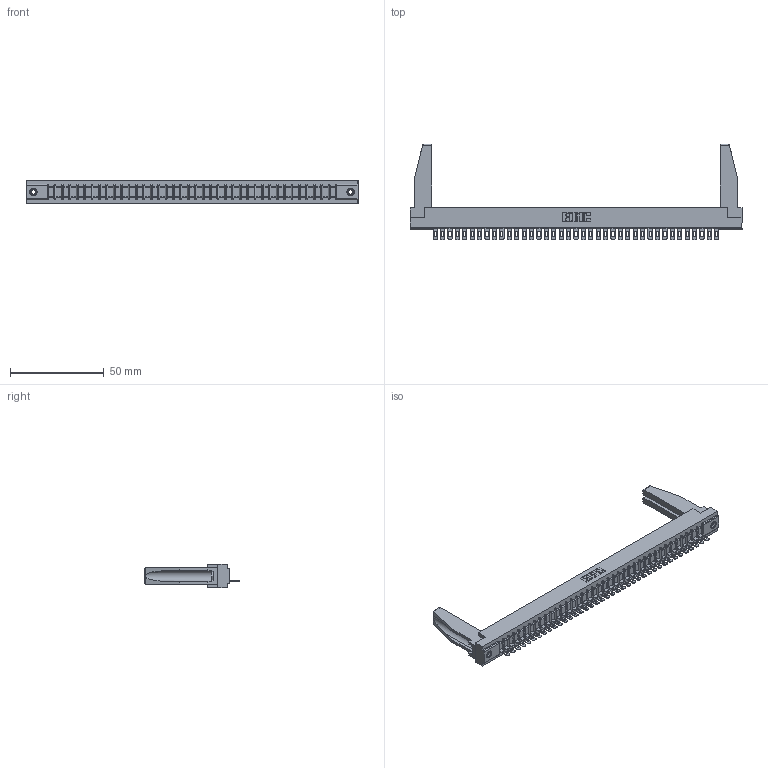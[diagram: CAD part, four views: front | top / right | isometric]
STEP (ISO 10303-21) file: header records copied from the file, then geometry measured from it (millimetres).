
FILE_DESCRIPTION (( 'STEP AP203' ), '1' );
FILE_NAME ('357-039-501-178.STEP', '2019-09-17T08:16:13', ( '' ), ( '' ), 'SwSTEP 2.0', 'SolidWorks 2016', '' );
FILE_SCHEMA (( 'CONFIG_CONTROL_DESIGN' ));
Length unit declared in the file: inch
Products named in the file (5): 307-220-078; 345-250-001_345-250-001-102; 307-290-002_501; 307 Part_.156 Dia Mounting Holes; 357-039-501-178
Assembly tree (44 placements, depth 2):
  357-039-501-178
    307 Part_.156 Dia Mounting Holes
    307-290-002_501  x39
    307-220-078  x2
    345-250-001_345-250-001-102  x2
Bounding box: 177.55 x 51.13 x 12.7 mm (x, y, z)
Volume: 23004.6 mm3; surface area: 27927 mm2
Topology: 44 solids, 44 shells, 3252 faces, 9935 edges, 6506 vertices
Faces by surface type: plane 1870, cylinder 1286, sphere 80, cone 12, torus 4
Entity records: 37037 total; most frequent: CARTESIAN_POINT 6246, ORIENTED_EDGE 6192, DIRECTION 6030, EDGE_CURVE 3096, LINE 2370, VECTOR 2370, VERTEX_POINT 2004, AXIS2_PLACEMENT_3D 1830
